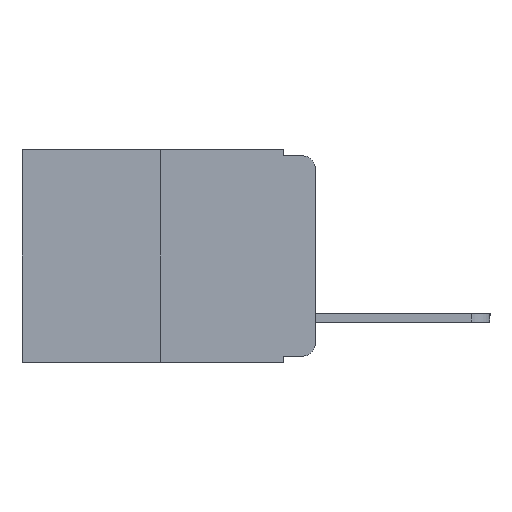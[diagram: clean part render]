
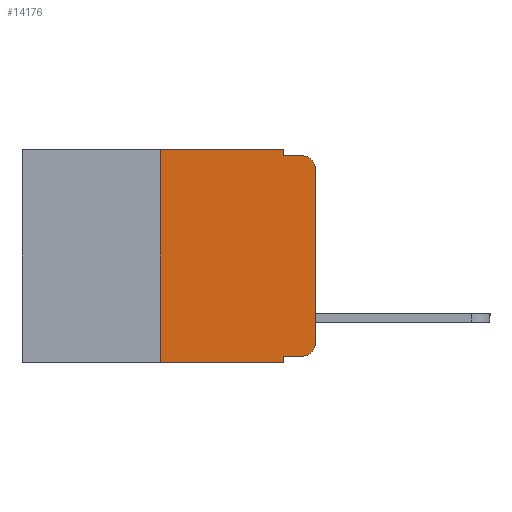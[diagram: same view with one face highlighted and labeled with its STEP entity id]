
A CAD part, left-side view. The second image highlights one B-rep face of the part: STEP entity #14176.
In plain terms, the highlighted planar face has unit normal (-1, 0, 0).
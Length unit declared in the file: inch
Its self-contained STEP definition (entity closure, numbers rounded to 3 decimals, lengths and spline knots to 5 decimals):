
#34 = DIRECTION ( 'NONE',  ( 0., -1., 0. ) ) ;
#228 = VECTOR ( 'NONE', #5967, 39.37008 ) ;
#266 = VERTEX_POINT ( 'NONE', #7939 ) ;
#272 = ORIENTED_EDGE ( 'NONE', *, *, #6724, .F. ) ;
#514 = VERTEX_POINT ( 'NONE', #19241 ) ;
#575 = CARTESIAN_POINT ( 'NONE',  ( 0., 0.051, -0.01 ) ) ;
#601 = CARTESIAN_POINT ( 'NONE',  ( 0., 0.02, -0.333 ) ) ;
#744 = CARTESIAN_POINT ( 'NONE',  ( 0., 0.473, 0. ) ) ;
#863 = VECTOR ( 'NONE', #19605, 39.37008 ) ;
#967 = CARTESIAN_POINT ( 'NONE',  ( 0., 0.02, -0.313 ) ) ;
#1051 = CARTESIAN_POINT ( 'NONE',  ( 0., 0., -0.313 ) ) ;
#1401 = VECTOR ( 'NONE', #5279, 39.37008 ) ;
#1892 = DIRECTION ( 'NONE',  ( 0., 0., 1. ) ) ;
#2234 = DIRECTION ( 'NONE',  ( 0., -1., 0. ) ) ;
#2550 = VERTEX_POINT ( 'NONE', #17224 ) ;
#2599 = DIRECTION ( 'NONE',  ( 0., 0., -1. ) ) ;
#2660 = LINE ( 'NONE', #10464, #10569 ) ;
#3752 = CARTESIAN_POINT ( 'NONE',  ( 0., 0.25, -0.343 ) ) ;
#4656 = LINE ( 'NONE', #15514, #863 ) ;
#5150 = LINE ( 'NONE', #575, #5625 ) ;
#5279 = DIRECTION ( 'NONE',  ( 0., 0., -1. ) ) ;
#5566 = PLANE ( 'NONE',  #13050 ) ;
#5625 = VECTOR ( 'NONE', #2234, 39.37008 ) ;
#5822 = LINE ( 'NONE', #6849, #1401 ) ;
#5900 = VERTEX_POINT ( 'NONE', #8635 ) ;
#5967 = DIRECTION ( 'NONE',  ( 0., -1., 0. ) ) ;
#6490 = CARTESIAN_POINT ( 'NONE',  ( 0., 0.473, 0. ) ) ;
#6526 = ORIENTED_EDGE ( 'NONE', *, *, #13099, .T. ) ;
#6532 = VERTEX_POINT ( 'NONE', #601 ) ;
#6724 = EDGE_CURVE ( 'NONE', #14688, #5900, #12362, .T. ) ;
#6849 = CARTESIAN_POINT ( 'NONE',  ( 0., 0.051, 0. ) ) ;
#7042 = ORIENTED_EDGE ( 'NONE', *, *, #12864, .T. ) ;
#7147 = DIRECTION ( 'NONE',  ( 1., 0., 0. ) ) ;
#7194 = CARTESIAN_POINT ( 'NONE',  ( 0., 0.02, -0.03 ) ) ;
#7939 = CARTESIAN_POINT ( 'NONE',  ( 0., 0., -0.03 ) ) ;
#8211 = DIRECTION ( 'NONE',  ( 0., 0., -1. ) ) ;
#8563 = CARTESIAN_POINT ( 'NONE',  ( 0., 0.25, 0. ) ) ;
#8635 = CARTESIAN_POINT ( 'NONE',  ( 0., 0.051, 0. ) ) ;
#8844 = DIRECTION ( 'NONE',  ( 0., 0., -1. ) ) ;
#9282 = VERTEX_POINT ( 'NONE', #1051 ) ;
#9535 = EDGE_CURVE ( 'NONE', #9648, #15726, #10815, .T. ) ;
#9648 = VERTEX_POINT ( 'NONE', #3752 ) ;
#9787 = ORIENTED_EDGE ( 'NONE', *, *, #9535, .T. ) ;
#10464 = CARTESIAN_POINT ( 'NONE',  ( 0., 0., 0. ) ) ;
#10517 = ORIENTED_EDGE ( 'NONE', *, *, #13366, .T. ) ;
#10569 = VECTOR ( 'NONE', #11986, 39.37008 ) ;
#10815 = LINE ( 'NONE', #15587, #13315 ) ;
#11464 = ORIENTED_EDGE ( 'NONE', *, *, #13247, .F. ) ;
#11498 = LINE ( 'NONE', #15699, #12412 ) ;
#11629 = CARTESIAN_POINT ( 'NONE',  ( 0., 0.051, -0.333 ) ) ;
#11736 = CIRCLE ( 'NONE', #11979, 0.02 ) ;
#11979 = AXIS2_PLACEMENT_3D ( 'NONE', #967, #12003, #2599 ) ;
#11986 = DIRECTION ( 'NONE',  ( 0., 0., 1. ) ) ;
#12003 = DIRECTION ( 'NONE',  ( -1., 0., 0. ) ) ;
#12362 = LINE ( 'NONE', #6490, #228 ) ;
#12412 = VECTOR ( 'NONE', #1892, 39.37008 ) ;
#12821 = ORIENTED_EDGE ( 'NONE', *, *, #13162, .F. ) ;
#12864 = EDGE_CURVE ( 'NONE', #6532, #9282, #11736, .T. ) ;
#13050 = AXIS2_PLACEMENT_3D ( 'NONE', #744, #7147, #17539 ) ;
#13099 = EDGE_CURVE ( 'NONE', #13782, #6532, #4656, .T. ) ;
#13153 = EDGE_CURVE ( 'NONE', #13782, #15726, #18605, .T. ) ;
#13162 = EDGE_CURVE ( 'NONE', #9648, #14688, #11498, .T. ) ;
#13163 = AXIS2_PLACEMENT_3D ( 'NONE', #7194, #17592, #8844 ) ;
#13217 = EDGE_CURVE ( 'NONE', #5900, #514, #5822, .T. ) ;
#13247 = EDGE_CURVE ( 'NONE', #514, #2550, #5150, .T. ) ;
#13312 = EDGE_CURVE ( 'NONE', #266, #2550, #19047, .T. ) ;
#13315 = VECTOR ( 'NONE', #34, 39.37008 ) ;
#13366 = EDGE_CURVE ( 'NONE', #9282, #266, #2660, .T. ) ;
#13782 = VERTEX_POINT ( 'NONE', #11629 ) ;
#14176 = ADVANCED_FACE ( 'NONE', ( #15818 ), #5566, .F. ) ;
#14688 = VERTEX_POINT ( 'NONE', #8563 ) ;
#14865 = ORIENTED_EDGE ( 'NONE', *, *, #13312, .T. ) ;
#14894 = VECTOR ( 'NONE', #8211, 39.37008 ) ;
#15318 = ORIENTED_EDGE ( 'NONE', *, *, #13217, .F. ) ;
#15514 = CARTESIAN_POINT ( 'NONE',  ( 0., 0.051, -0.333 ) ) ;
#15587 = CARTESIAN_POINT ( 'NONE',  ( 0., 0.473, -0.343 ) ) ;
#15649 = CARTESIAN_POINT ( 'NONE',  ( 0., 0.051, 0. ) ) ;
#15699 = CARTESIAN_POINT ( 'NONE',  ( 0., 0.25, 0. ) ) ;
#15726 = VERTEX_POINT ( 'NONE', #17208 ) ;
#15818 = FACE_OUTER_BOUND ( 'NONE', #17293, .T. ) ;
#17208 = CARTESIAN_POINT ( 'NONE',  ( 0., 0.051, -0.343 ) ) ;
#17224 = CARTESIAN_POINT ( 'NONE',  ( 0., 0.02, -0.01 ) ) ;
#17293 = EDGE_LOOP ( 'NONE', ( #10517, #14865, #11464, #15318, #272, #12821, #9787, #17517, #6526, #7042 ) ) ;
#17517 = ORIENTED_EDGE ( 'NONE', *, *, #13153, .F. ) ;
#17539 = DIRECTION ( 'NONE',  ( 0., 0., -1. ) ) ;
#17592 = DIRECTION ( 'NONE',  ( -1., 0., 0. ) ) ;
#18605 = LINE ( 'NONE', #15649, #14894 ) ;
#19047 = CIRCLE ( 'NONE', #13163, 0.02 ) ;
#19241 = CARTESIAN_POINT ( 'NONE',  ( 0., 0.051, -0.01 ) ) ;
#19605 = DIRECTION ( 'NONE',  ( 0., -1., 0. ) ) ;
